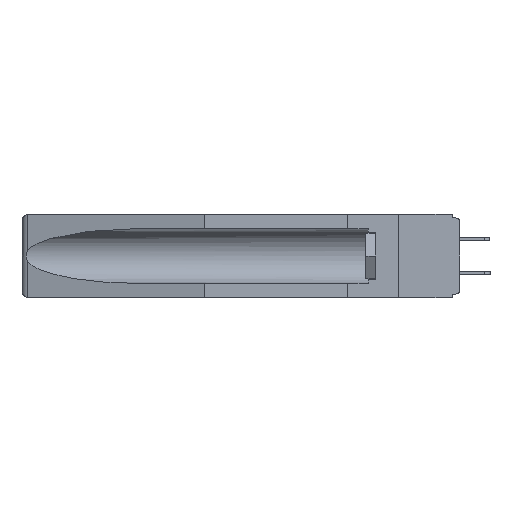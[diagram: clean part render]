
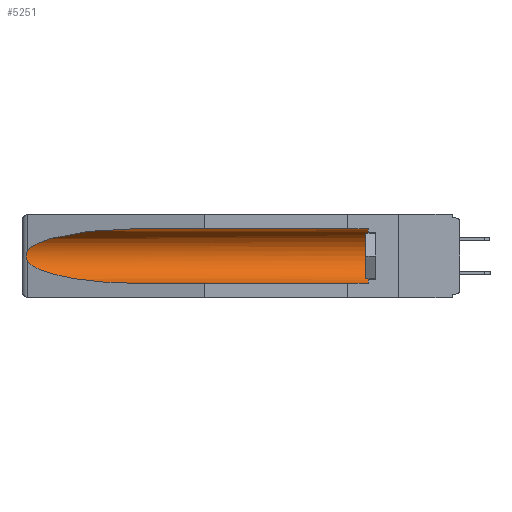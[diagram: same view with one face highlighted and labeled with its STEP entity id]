
A CAD part, left-side view. The second image highlights one B-rep face of the part: STEP entity #5251.
In plain terms, the highlighted cylindrical face has radius 2.857 mm (diameter 5.715 mm), a partial arc.
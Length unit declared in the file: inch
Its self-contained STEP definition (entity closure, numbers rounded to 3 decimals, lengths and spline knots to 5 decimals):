
#85 = CARTESIAN_POINT ( 'NONE',  ( 0.155, -0.30754, -0.059 ) ) ;
#410 = ORIENTED_EDGE ( 'NONE', *, *, #13152, .T. ) ;
#430 = AXIS2_PLACEMENT_3D ( 'NONE', #19465, #17201, #5540 ) ;
#800 = B_SPLINE_CURVE_WITH_KNOTS ( 'NONE', 3,
 ( #2950, #24917, #22803, #16791, #14939, #9121, #14685, #1045, #20926, #12682 ),
 .UNSPECIFIED., .F., .F.,
 ( 4, 2, 2, 2, 4 ),
 ( 0., 0.00029, 0.00058, 0.00087, 0.00117 ),
 .UNSPECIFIED. ) ;
#844 = FACE_OUTER_BOUND ( 'NONE', #9179, .T. ) ;
#1045 = CARTESIAN_POINT ( 'NONE',  ( 0.26655, 1.53094, -0.18657 ) ) ;
#1732 = CARTESIAN_POINT ( 'NONE',  ( 0.155, 1.07973, -0.059 ) ) ;
#2479 = VERTEX_POINT ( 'NONE', #13290 ) ;
#2950 = CARTESIAN_POINT ( 'NONE',  ( 0.26537, 1.52718, -0.14972 ) ) ;
#4595 = AXIS2_PLACEMENT_3D ( 'NONE', #16502, #16332, #4831 ) ;
#4831 = DIRECTION ( 'NONE',  ( 0., 0., 1. ) ) ;
#5206 = VERTEX_POINT ( 'NONE', #9163 ) ;
#5251 = ADVANCED_FACE ( 'NONE', ( #844 ), #5459, .F. ) ;
#5415 = EDGE_CURVE ( 'NONE', #2479, #8779, #17601, .T. ) ;
#5459 = CYLINDRICAL_SURFACE ( 'NONE', #430, 0.1125 ) ;
#5540 = DIRECTION ( 'NONE',  ( 0., 0., 1. ) ) ;
#5591 = VERTEX_POINT ( 'NONE', #10900 ) ;
#6117 = CARTESIAN_POINT ( 'NONE',  ( 0.26537, 1.52718, -0.14972 ) ) ;
#6515 =( BOUNDED_CURVE ( )  B_SPLINE_CURVE ( 3, ( #15308, #9216, #13442, #11208 ),
 .UNSPECIFIED., .F., .F. ) 
 B_SPLINE_CURVE_WITH_KNOTS ( ( 4, 4 ),
 ( 0.1948, 1.5708 ),
 .UNSPECIFIED. ) 
 CURVE ( )  GEOMETRIC_REPRESENTATION_ITEM ( )  RATIONAL_B_SPLINE_CURVE ( ( 1., 0.848, 0.848, 1. ) ) 
 REPRESENTATION_ITEM ( '' )  );
#7397 = CARTESIAN_POINT ( 'NONE',  ( 0.21114, 1.30732, -0.059 ) ) ;
#7885 = EDGE_CURVE ( 'NONE', #5206, #2479, #15853, .T. ) ;
#8067 = LINE ( 'NONE', #11272, #10230 ) ;
#8779 = VERTEX_POINT ( 'NONE', #6117 ) ;
#9017 = EDGE_CURVE ( 'NONE', #5591, #10141, #6515, .T. ) ;
#9076 = CARTESIAN_POINT ( 'NONE',  ( 0.155, 1.07973, -0.284 ) ) ;
#9121 = CARTESIAN_POINT ( 'NONE',  ( 0.2675, 1.53308, -0.17534 ) ) ;
#9163 = CARTESIAN_POINT ( 'NONE',  ( 0.155, 0.126, -0.059 ) ) ;
#9179 = EDGE_LOOP ( 'NONE', ( #13757, #410, #15927, #10914, #15741, #20112 ) ) ;
#9216 = CARTESIAN_POINT ( 'NONE',  ( 0.25451, 1.48313, -0.24835 ) ) ;
#9720 = DIRECTION ( 'NONE',  ( 0., 1., 0. ) ) ;
#10141 = VERTEX_POINT ( 'NONE', #9076 ) ;
#10230 = VECTOR ( 'NONE', #15280, 39.37008 ) ;
#10567 = CARTESIAN_POINT ( 'NONE',  ( 0.155, 0.126, -0.284 ) ) ;
#10900 = CARTESIAN_POINT ( 'NONE',  ( 0.26537, 1.52718, -0.19328 ) ) ;
#10914 = ORIENTED_EDGE ( 'NONE', *, *, #22391, .F. ) ;
#11208 = CARTESIAN_POINT ( 'NONE',  ( 0.155, 1.07973, -0.284 ) ) ;
#11272 = CARTESIAN_POINT ( 'NONE',  ( 0.155, -0.30754, -0.284 ) ) ;
#12682 = CARTESIAN_POINT ( 'NONE',  ( 0.26537, 1.52718, -0.19328 ) ) ;
#13152 = EDGE_CURVE ( 'NONE', #8779, #5591, #800, .T. ) ;
#13290 = CARTESIAN_POINT ( 'NONE',  ( 0.155, 1.07973, -0.059 ) ) ;
#13442 = CARTESIAN_POINT ( 'NONE',  ( 0.21114, 1.30732, -0.284 ) ) ;
#13757 = ORIENTED_EDGE ( 'NONE', *, *, #5415, .T. ) ;
#14299 = CIRCLE ( 'NONE', #4595, 0.1125 ) ;
#14685 = CARTESIAN_POINT ( 'NONE',  ( 0.2673, 1.53269, -0.17917 ) ) ;
#14939 = CARTESIAN_POINT ( 'NONE',  ( 0.2675, 1.53308, -0.16763 ) ) ;
#15280 = DIRECTION ( 'NONE',  ( 0., 1., 0. ) ) ;
#15308 = CARTESIAN_POINT ( 'NONE',  ( 0.26537, 1.52718, -0.19328 ) ) ;
#15741 = ORIENTED_EDGE ( 'NONE', *, *, #18834, .T. ) ;
#15853 = LINE ( 'NONE', #85, #23982 ) ;
#15907 = CARTESIAN_POINT ( 'NONE',  ( 0.26537, 1.52718, -0.14972 ) ) ;
#15927 = ORIENTED_EDGE ( 'NONE', *, *, #9017, .T. ) ;
#16332 = DIRECTION ( 'NONE',  ( 0., -1., 0. ) ) ;
#16502 = CARTESIAN_POINT ( 'NONE',  ( 0.155, 0.126, -0.1715 ) ) ;
#16791 = CARTESIAN_POINT ( 'NONE',  ( 0.2673, 1.5327, -0.16383 ) ) ;
#17201 = DIRECTION ( 'NONE',  ( 0., 1., 0. ) ) ;
#17601 =( BOUNDED_CURVE ( )  B_SPLINE_CURVE ( 3, ( #1732, #7397, #17922, #15907 ),
 .UNSPECIFIED., .F., .F. ) 
 B_SPLINE_CURVE_WITH_KNOTS ( ( 4, 4 ),
 ( 4.71239, 6.08839 ),
 .UNSPECIFIED. ) 
 CURVE ( )  GEOMETRIC_REPRESENTATION_ITEM ( )  RATIONAL_B_SPLINE_CURVE ( ( 1., 0.848, 0.848, 1. ) ) 
 REPRESENTATION_ITEM ( '' )  );
#17922 = CARTESIAN_POINT ( 'NONE',  ( 0.25451, 1.48313, -0.09465 ) ) ;
#18834 = EDGE_CURVE ( 'NONE', #22146, #5206, #14299, .T. ) ;
#19465 = CARTESIAN_POINT ( 'NONE',  ( 0.155, -0.30754, -0.1715 ) ) ;
#20112 = ORIENTED_EDGE ( 'NONE', *, *, #7885, .T. ) ;
#20926 = CARTESIAN_POINT ( 'NONE',  ( 0.26597, 1.5296, -0.19026 ) ) ;
#22146 = VERTEX_POINT ( 'NONE', #10567 ) ;
#22391 = EDGE_CURVE ( 'NONE', #22146, #10141, #8067, .T. ) ;
#22803 = CARTESIAN_POINT ( 'NONE',  ( 0.26654, 1.53092, -0.15636 ) ) ;
#23982 = VECTOR ( 'NONE', #9720, 39.37008 ) ;
#24917 = CARTESIAN_POINT ( 'NONE',  ( 0.26597, 1.52961, -0.15275 ) ) ;
